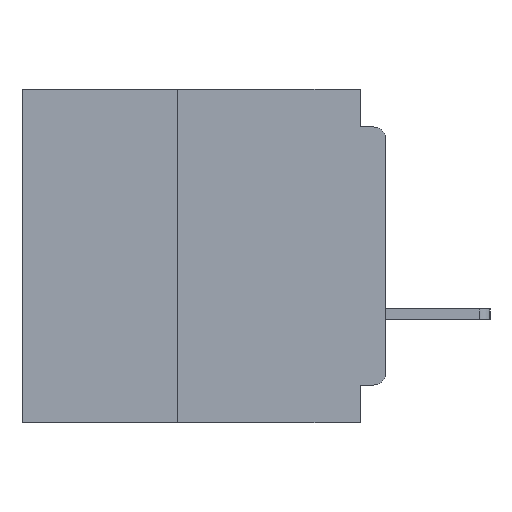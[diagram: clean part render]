
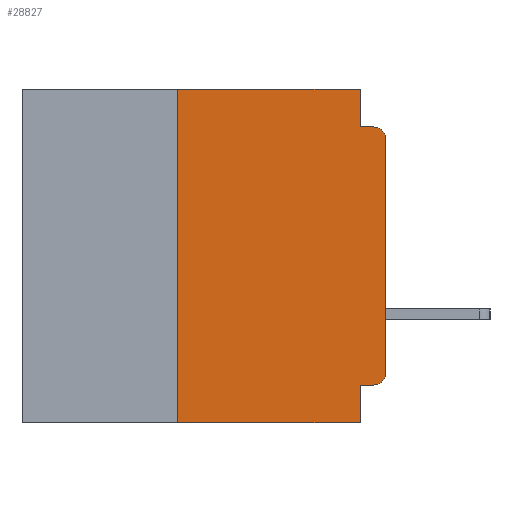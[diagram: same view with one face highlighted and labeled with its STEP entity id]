
A CAD part, left-side view. The second image highlights one B-rep face of the part: STEP entity #28827.
In plain terms, the highlighted planar face has unit normal (-1, 0, 0).
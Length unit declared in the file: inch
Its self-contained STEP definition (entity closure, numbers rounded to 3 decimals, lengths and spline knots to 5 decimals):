
#856 = VECTOR ( 'NONE', #53712, 39.37008 ) ;
#2216 = LINE ( 'NONE', #20597, #856 ) ;
#4528 = AXIS2_PLACEMENT_3D ( 'NONE', #41368, #16409, #49716 ) ;
#4810 = LINE ( 'NONE', #26074, #15872 ) ;
#5000 = CARTESIAN_POINT ( 'NONE',  ( 0., 0.031, -0.355 ) ) ;
#5378 = LINE ( 'NONE', #23606, #27447 ) ;
#5411 = DIRECTION ( 'NONE',  ( 0., 0., 1. ) ) ;
#5509 = CARTESIAN_POINT ( 'NONE',  ( 0., 0.015, -0.06 ) ) ;
#7882 = VERTEX_POINT ( 'NONE', #18582 ) ;
#8291 = VECTOR ( 'NONE', #28445, 39.37008 ) ;
#8631 = EDGE_LOOP ( 'NONE', ( #44823, #15783, #25706, #9389, #9572, #44588, #28113, #16599, #44084, #24364 ) ) ;
#9389 = ORIENTED_EDGE ( 'NONE', *, *, #46097, .F. ) ;
#9572 = ORIENTED_EDGE ( 'NONE', *, *, #51519, .F. ) ;
#9692 = DIRECTION ( 'NONE',  ( 0., 0., -1. ) ) ;
#10273 = VERTEX_POINT ( 'NONE', #35717 ) ;
#10447 = EDGE_CURVE ( 'NONE', #48161, #10273, #17294, .T. ) ;
#10996 = CARTESIAN_POINT ( 'NONE',  ( 0., 0.015, -0.355 ) ) ;
#11068 = CARTESIAN_POINT ( 'NONE',  ( 0., 0.25, -0.4 ) ) ;
#11718 = FACE_OUTER_BOUND ( 'NONE', #8631, .T. ) ;
#12386 = CARTESIAN_POINT ( 'NONE',  ( 0., 0.031, -0.045 ) ) ;
#13300 = VERTEX_POINT ( 'NONE', #43153 ) ;
#15738 = LINE ( 'NONE', #49643, #36487 ) ;
#15783 = ORIENTED_EDGE ( 'NONE', *, *, #27107, .T. ) ;
#15872 = VECTOR ( 'NONE', #5411, 39.37008 ) ;
#16409 = DIRECTION ( 'NONE',  ( 1., 0., 0. ) ) ;
#16599 = ORIENTED_EDGE ( 'NONE', *, *, #26709, .F. ) ;
#17294 = CIRCLE ( 'NONE', #44420, 0.015 ) ;
#17742 = EDGE_CURVE ( 'NONE', #45579, #18784, #53193, .T. ) ;
#17807 = VERTEX_POINT ( 'NONE', #11068 ) ;
#18582 = CARTESIAN_POINT ( 'NONE',  ( 0., 0.031, 0. ) ) ;
#18784 = VERTEX_POINT ( 'NONE', #30052 ) ;
#18846 = CARTESIAN_POINT ( 'NONE',  ( 0., 0., -0.045 ) ) ;
#19728 = VECTOR ( 'NONE', #36955, 39.37008 ) ;
#20159 = VECTOR ( 'NONE', #23004, 39.37008 ) ;
#20454 = CARTESIAN_POINT ( 'NONE',  ( 0., 0.015, -0.34 ) ) ;
#20597 = CARTESIAN_POINT ( 'NONE',  ( 0., 0., -0.355 ) ) ;
#23004 = DIRECTION ( 'NONE',  ( 0., -1., 0. ) ) ;
#23606 = CARTESIAN_POINT ( 'NONE',  ( 0., 0.437, 0. ) ) ;
#24279 = CARTESIAN_POINT ( 'NONE',  ( 0., 0.031, 0. ) ) ;
#24364 = ORIENTED_EDGE ( 'NONE', *, *, #10447, .T. ) ;
#24650 = DIRECTION ( 'NONE',  ( 0., 0., -1. ) ) ;
#25021 = VERTEX_POINT ( 'NONE', #5000 ) ;
#25706 = ORIENTED_EDGE ( 'NONE', *, *, #17742, .F. ) ;
#26074 = CARTESIAN_POINT ( 'NONE',  ( 0., 0.25, -0.4 ) ) ;
#26709 = EDGE_CURVE ( 'NONE', #25021, #36498, #28815, .T. ) ;
#27107 = EDGE_CURVE ( 'NONE', #41561, #18784, #31350, .T. ) ;
#27447 = VECTOR ( 'NONE', #52553, 39.37008 ) ;
#28113 = ORIENTED_EDGE ( 'NONE', *, *, #32273, .T. ) ;
#28445 = DIRECTION ( 'NONE',  ( 0., 0., -1. ) ) ;
#28815 = LINE ( 'NONE', #30032, #49526 ) ;
#28827 = ADVANCED_FACE ( 'NONE', ( #11718 ), #45518, .F. ) ;
#30032 = CARTESIAN_POINT ( 'NONE',  ( 0., 0.031, -0.4 ) ) ;
#30052 = CARTESIAN_POINT ( 'NONE',  ( 0., 0.015, -0.045 ) ) ;
#30620 = CARTESIAN_POINT ( 'NONE',  ( 0., 0., -0.06 ) ) ;
#31350 = CIRCLE ( 'NONE', #32984, 0.015 ) ;
#32058 = LINE ( 'NONE', #32789, #19728 ) ;
#32273 = EDGE_CURVE ( 'NONE', #17807, #36498, #32058, .T. ) ;
#32661 = EDGE_CURVE ( 'NONE', #48161, #25021, #2216, .T. ) ;
#32789 = CARTESIAN_POINT ( 'NONE',  ( 0., 0.437, -0.4 ) ) ;
#32984 = AXIS2_PLACEMENT_3D ( 'NONE', #5509, #34503, #9692 ) ;
#34187 = DIRECTION ( 'NONE',  ( 0., 0., -1. ) ) ;
#34503 = DIRECTION ( 'NONE',  ( -1., 0., 0. ) ) ;
#35717 = CARTESIAN_POINT ( 'NONE',  ( 0., 0., -0.34 ) ) ;
#36487 = VECTOR ( 'NONE', #45274, 39.37008 ) ;
#36498 = VERTEX_POINT ( 'NONE', #45665 ) ;
#36955 = DIRECTION ( 'NONE',  ( 0., -1., 0. ) ) ;
#41327 = LINE ( 'NONE', #24279, #8291 ) ;
#41368 = CARTESIAN_POINT ( 'NONE',  ( 0., 0.437, 0. ) ) ;
#41561 = VERTEX_POINT ( 'NONE', #30620 ) ;
#43153 = CARTESIAN_POINT ( 'NONE',  ( 0., 0.25, 0. ) ) ;
#43347 = EDGE_CURVE ( 'NONE', #17807, #13300, #4810, .T. ) ;
#44084 = ORIENTED_EDGE ( 'NONE', *, *, #32661, .F. ) ;
#44420 = AXIS2_PLACEMENT_3D ( 'NONE', #20454, #49430, #24650 ) ;
#44588 = ORIENTED_EDGE ( 'NONE', *, *, #43347, .F. ) ;
#44823 = ORIENTED_EDGE ( 'NONE', *, *, #49013, .T. ) ;
#45274 = DIRECTION ( 'NONE',  ( 0., 0., 1. ) ) ;
#45518 = PLANE ( 'NONE',  #4528 ) ;
#45579 = VERTEX_POINT ( 'NONE', #12386 ) ;
#45665 = CARTESIAN_POINT ( 'NONE',  ( 0., 0.031, -0.4 ) ) ;
#46097 = EDGE_CURVE ( 'NONE', #7882, #45579, #41327, .T. ) ;
#48161 = VERTEX_POINT ( 'NONE', #10996 ) ;
#49013 = EDGE_CURVE ( 'NONE', #10273, #41561, #15738, .T. ) ;
#49430 = DIRECTION ( 'NONE',  ( -1., 0., 0. ) ) ;
#49526 = VECTOR ( 'NONE', #34187, 39.37008 ) ;
#49643 = CARTESIAN_POINT ( 'NONE',  ( 0., 0., 0. ) ) ;
#49716 = DIRECTION ( 'NONE',  ( 0., 0., -1. ) ) ;
#51519 = EDGE_CURVE ( 'NONE', #13300, #7882, #5378, .T. ) ;
#52553 = DIRECTION ( 'NONE',  ( 0., -1., 0. ) ) ;
#53193 = LINE ( 'NONE', #18846, #20159 ) ;
#53712 = DIRECTION ( 'NONE',  ( 0., 1., 0. ) ) ;
